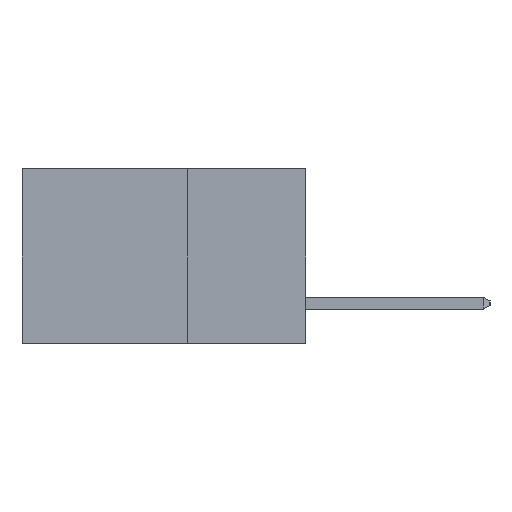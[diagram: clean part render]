
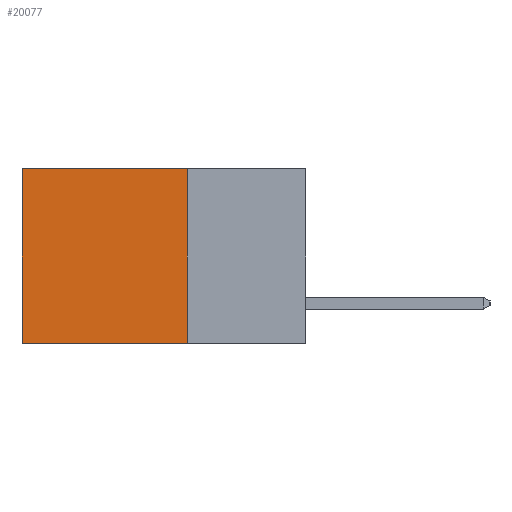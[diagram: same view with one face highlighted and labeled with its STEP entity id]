
A CAD part, left-side view. The second image highlights one B-rep face of the part: STEP entity #20077.
In plain terms, the highlighted planar face has unit normal (-1, 0, 0).
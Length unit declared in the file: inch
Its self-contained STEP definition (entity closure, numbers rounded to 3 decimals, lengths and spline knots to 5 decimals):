
#297 = CARTESIAN_POINT ( 'NONE',  ( 0.2615, 0.25, -0.37 ) ) ;
#374 = CARTESIAN_POINT ( 'NONE',  ( 0.2615, 0.25, 0. ) ) ;
#635 = CARTESIAN_POINT ( 'NONE',  ( 0.2615, 0.25, -0.37 ) ) ;
#1093 = ORIENTED_EDGE ( 'NONE', *, *, #21217, .F. ) ;
#1166 = VERTEX_POINT ( 'NONE', #374 ) ;
#1756 = DIRECTION ( 'NONE',  ( 0., 1., 0. ) ) ;
#1888 = VECTOR ( 'NONE', #1756, 39.37008 ) ;
#2241 = CARTESIAN_POINT ( 'NONE',  ( 0.2615, 0.25, -0.37 ) ) ;
#2275 = DIRECTION ( 'NONE',  ( 0., 0., -1. ) ) ;
#3049 = VECTOR ( 'NONE', #2275, 39.37008 ) ;
#3670 = LINE ( 'NONE', #297, #3049 ) ;
#4023 = PLANE ( 'NONE',  #6753 ) ;
#4537 = CARTESIAN_POINT ( 'NONE',  ( 0.2615, 0.6, 0. ) ) ;
#4910 = VECTOR ( 'NONE', #17582, 39.37008 ) ;
#5068 = ORIENTED_EDGE ( 'NONE', *, *, #17968, .T. ) ;
#5971 = CARTESIAN_POINT ( 'NONE',  ( 0.2615, 0.25, -0.37 ) ) ;
#6254 = LINE ( 'NONE', #22000, #11769 ) ;
#6753 = AXIS2_PLACEMENT_3D ( 'NONE', #5971, #18932, #7837 ) ;
#7837 = DIRECTION ( 'NONE',  ( 0., 0., -1. ) ) ;
#8404 = VERTEX_POINT ( 'NONE', #22186 ) ;
#8415 = EDGE_CURVE ( 'NONE', #15992, #8404, #6254, .T. ) ;
#9911 = LINE ( 'NONE', #635, #4910 ) ;
#10018 = FACE_OUTER_BOUND ( 'NONE', #15200, .T. ) ;
#10381 = VERTEX_POINT ( 'NONE', #2241 ) ;
#10477 = EDGE_CURVE ( 'NONE', #10381, #8404, #9911, .T. ) ;
#11295 = LINE ( 'NONE', #22106, #1888 ) ;
#11769 = VECTOR ( 'NONE', #22059, 39.37008 ) ;
#15200 = EDGE_LOOP ( 'NONE', ( #19766, #17353, #1093, #5068 ) ) ;
#15992 = VERTEX_POINT ( 'NONE', #4537 ) ;
#17353 = ORIENTED_EDGE ( 'NONE', *, *, #10477, .F. ) ;
#17582 = DIRECTION ( 'NONE',  ( 0., 1., 0. ) ) ;
#17968 = EDGE_CURVE ( 'NONE', #1166, #15992, #11295, .T. ) ;
#18932 = DIRECTION ( 'NONE',  ( 1., 0., 0. ) ) ;
#19766 = ORIENTED_EDGE ( 'NONE', *, *, #8415, .T. ) ;
#20077 = ADVANCED_FACE ( 'NONE', ( #10018 ), #4023, .F. ) ;
#21217 = EDGE_CURVE ( 'NONE', #1166, #10381, #3670, .T. ) ;
#22000 = CARTESIAN_POINT ( 'NONE',  ( 0.2615, 0.6, -0.37 ) ) ;
#22059 = DIRECTION ( 'NONE',  ( 0., 0., -1. ) ) ;
#22106 = CARTESIAN_POINT ( 'NONE',  ( 0.2615, 0.25, 0. ) ) ;
#22186 = CARTESIAN_POINT ( 'NONE',  ( 0.2615, 0.6, -0.37 ) ) ;
